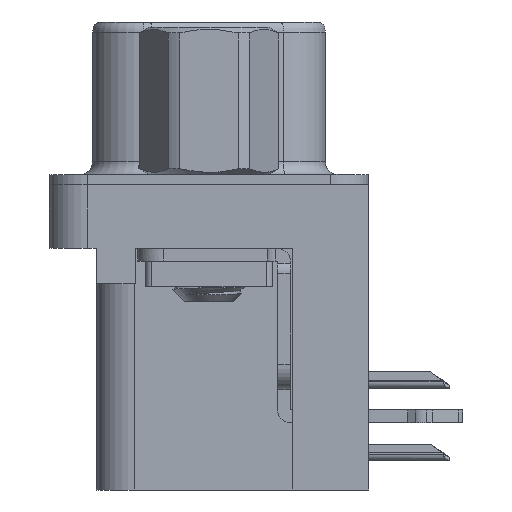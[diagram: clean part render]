
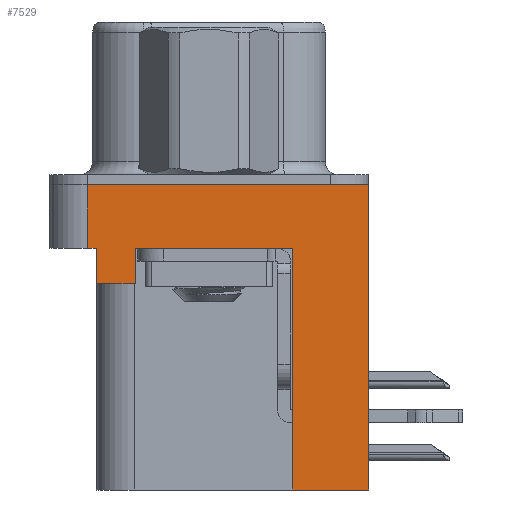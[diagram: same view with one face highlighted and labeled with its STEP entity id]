
A CAD part, left-side view. The second image highlights one B-rep face of the part: STEP entity #7529.
In plain terms, the highlighted planar face has unit normal (-1, 0, 0).
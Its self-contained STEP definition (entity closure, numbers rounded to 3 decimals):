
#547 = DIRECTION ( 'NONE',  ( 0., -1., 0. ) ) ;
#776 = CARTESIAN_POINT ( 'NONE',  ( -2.91, -3.295, -2.5 ) ) ;
#987 = ORIENTED_EDGE ( 'NONE', *, *, #10293, .F. ) ;
#1171 = CARTESIAN_POINT ( 'NONE',  ( -2.91, -6.275, -2.5 ) ) ;
#1423 = CARTESIAN_POINT ( 'NONE',  ( -2.91, -3.295, -12. ) ) ;
#1904 = ORIENTED_EDGE ( 'NONE', *, *, #9725, .F. ) ;
#2155 = VECTOR ( 'NONE', #19515, 1000. ) ;
#2307 = CARTESIAN_POINT ( 'NONE',  ( -2.91, 4.425, -2.5 ) ) ;
#2386 = LINE ( 'NONE', #30779, #32310 ) ;
#2527 = ORIENTED_EDGE ( 'NONE', *, *, #4803, .T. ) ;
#2598 = DIRECTION ( 'NONE',  ( 0., 1., 0. ) ) ;
#3147 = EDGE_CURVE ( 'NONE', #25483, #13168, #7087, .T. ) ;
#3607 = EDGE_CURVE ( 'NONE', #25483, #7533, #6263, .T. ) ;
#3649 = DIRECTION ( 'NONE',  ( 0., 0., 1. ) ) ;
#4803 = EDGE_CURVE ( 'NONE', #7033, #4984, #20664, .T. ) ;
#4889 = EDGE_CURVE ( 'NONE', #22520, #11378, #6174, .T. ) ;
#4984 = VERTEX_POINT ( 'NONE', #2307 ) ;
#5751 = VECTOR ( 'NONE', #11542, 1000. ) ;
#6174 = LINE ( 'NONE', #24157, #5751 ) ;
#6263 = LINE ( 'NONE', #21574, #25464 ) ;
#6295 = FACE_OUTER_BOUND ( 'NONE', #24379, .T. ) ;
#6593 = DIRECTION ( 'NONE',  ( 0., 0., 1. ) ) ;
#6860 = CARTESIAN_POINT ( 'NONE',  ( -2.91, -6.275, -2.5 ) ) ;
#7033 = VERTEX_POINT ( 'NONE', #25712 ) ;
#7087 = LINE ( 'NONE', #22869, #11379 ) ;
#7529 = ADVANCED_FACE ( 'NONE', ( #6295 ), #29785, .T. ) ;
#7533 = VERTEX_POINT ( 'NONE', #13546 ) ;
#7730 = CARTESIAN_POINT ( 'NONE',  ( -2.91, -3.295, -12. ) ) ;
#8334 = LINE ( 'NONE', #25739, #18520 ) ;
#8643 = ORIENTED_EDGE ( 'NONE', *, *, #4889, .T. ) ;
#8800 = CARTESIAN_POINT ( 'NONE',  ( -2.91, -3.295, -12. ) ) ;
#8942 = VECTOR ( 'NONE', #9298, 1000. ) ;
#9298 = DIRECTION ( 'NONE',  ( 0., -1., 0. ) ) ;
#9725 = EDGE_CURVE ( 'NONE', #13168, #4984, #11859, .T. ) ;
#10293 = EDGE_CURVE ( 'NONE', #23645, #11378, #8334, .T. ) ;
#11378 = VERTEX_POINT ( 'NONE', #24984 ) ;
#11379 = VECTOR ( 'NONE', #2598, 1000. ) ;
#11542 = DIRECTION ( 'NONE',  ( 0., 0., 1. ) ) ;
#11781 = ORIENTED_EDGE ( 'NONE', *, *, #13016, .F. ) ;
#11859 = LINE ( 'NONE', #17899, #20833 ) ;
#13016 = EDGE_CURVE ( 'NONE', #27449, #13625, #25064, .T. ) ;
#13168 = VERTEX_POINT ( 'NONE', #19311 ) ;
#13546 = CARTESIAN_POINT ( 'NONE',  ( -2.91, 2.895, -2.5 ) ) ;
#13625 = VERTEX_POINT ( 'NONE', #776 ) ;
#13854 = DIRECTION ( 'NONE',  ( 0., 1., 0. ) ) ;
#15584 = ORIENTED_EDGE ( 'NONE', *, *, #30843, .F. ) ;
#16737 = LINE ( 'NONE', #1171, #2155 ) ;
#17475 = ORIENTED_EDGE ( 'NONE', *, *, #3607, .T. ) ;
#17899 = CARTESIAN_POINT ( 'NONE',  ( -2.91, 4.425, -3.9 ) ) ;
#18520 = VECTOR ( 'NONE', #547, 1000. ) ;
#19311 = CARTESIAN_POINT ( 'NONE',  ( -2.91, 4.425, -3.9 ) ) ;
#19515 = DIRECTION ( 'NONE',  ( 0., -1., 0. ) ) ;
#19570 = VECTOR ( 'NONE', #28531, 1000. ) ;
#20664 = LINE ( 'NONE', #6860, #8942 ) ;
#20833 = VECTOR ( 'NONE', #25429, 1000. ) ;
#21146 = EDGE_CURVE ( 'NONE', #7533, #13625, #16737, .T. ) ;
#21574 = CARTESIAN_POINT ( 'NONE',  ( -2.91, 2.895, -3.9 ) ) ;
#22520 = VERTEX_POINT ( 'NONE', #31947 ) ;
#22869 = CARTESIAN_POINT ( 'NONE',  ( -2.91, 4.425, -3.9 ) ) ;
#23250 = DIRECTION ( 'NONE',  ( 0., 0., 1. ) ) ;
#23645 = VERTEX_POINT ( 'NONE', #32293 ) ;
#24003 = VECTOR ( 'NONE', #13854, 1000. ) ;
#24073 = AXIS2_PLACEMENT_3D ( 'NONE', #31264, #28595, #3649 ) ;
#24157 = CARTESIAN_POINT ( 'NONE',  ( -2.91, -6.275, -2.5 ) ) ;
#24379 = EDGE_LOOP ( 'NONE', ( #987, #31256, #2527, #1904, #28582, #17475, #27356, #11781, #15584, #8643 ) ) ;
#24984 = CARTESIAN_POINT ( 'NONE',  ( -2.91, -6.275, 0. ) ) ;
#25064 = LINE ( 'NONE', #8800, #19570 ) ;
#25429 = DIRECTION ( 'NONE',  ( 0., 0., 1. ) ) ;
#25464 = VECTOR ( 'NONE', #6593, 1000. ) ;
#25483 = VERTEX_POINT ( 'NONE', #27811 ) ;
#25712 = CARTESIAN_POINT ( 'NONE',  ( -2.91, 4.775, -2.5 ) ) ;
#25739 = CARTESIAN_POINT ( 'NONE',  ( -2.91, -6.275, 0. ) ) ;
#27356 = ORIENTED_EDGE ( 'NONE', *, *, #21146, .T. ) ;
#27449 = VERTEX_POINT ( 'NONE', #7730 ) ;
#27811 = CARTESIAN_POINT ( 'NONE',  ( -2.91, 2.895, -3.9 ) ) ;
#28531 = DIRECTION ( 'NONE',  ( 0., 0., 1. ) ) ;
#28582 = ORIENTED_EDGE ( 'NONE', *, *, #3147, .F. ) ;
#28595 = DIRECTION ( 'NONE',  ( -1., 0., 0. ) ) ;
#29785 = PLANE ( 'NONE',  #24073 ) ;
#30779 = CARTESIAN_POINT ( 'NONE',  ( -2.91, 4.775, -2.5 ) ) ;
#30843 = EDGE_CURVE ( 'NONE', #22520, #27449, #32350, .T. ) ;
#31256 = ORIENTED_EDGE ( 'NONE', *, *, #31491, .F. ) ;
#31264 = CARTESIAN_POINT ( 'NONE',  ( -2.91, -6.275, -2.5 ) ) ;
#31491 = EDGE_CURVE ( 'NONE', #7033, #23645, #2386, .T. ) ;
#31947 = CARTESIAN_POINT ( 'NONE',  ( -2.91, -6.275, -12. ) ) ;
#32293 = CARTESIAN_POINT ( 'NONE',  ( -2.91, 4.775, 0. ) ) ;
#32310 = VECTOR ( 'NONE', #23250, 1000. ) ;
#32350 = LINE ( 'NONE', #1423, #24003 ) ;
